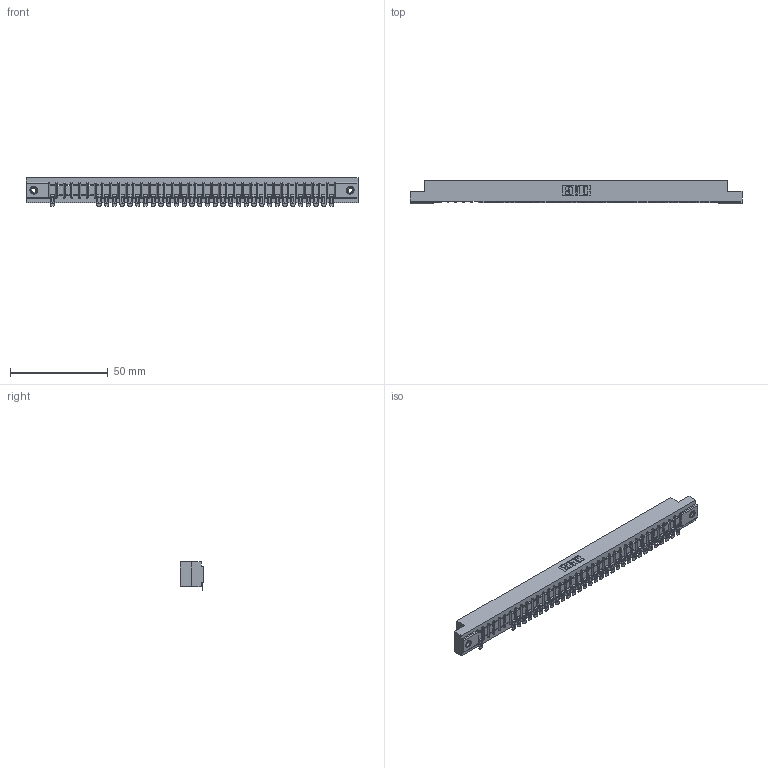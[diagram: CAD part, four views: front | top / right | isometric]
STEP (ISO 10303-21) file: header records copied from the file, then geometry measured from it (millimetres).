
FILE_DESCRIPTION (( 'STEP AP203' ), '1' );
FILE_NAME ('357-037-554-108.STEP', '2018-08-10T08:06:43', ( '' ), ( '' ), 'SwSTEP 2.0', 'SolidWorks 2016', '' );
FILE_SCHEMA (( 'CONFIG_CONTROL_DESIGN' ));
Length unit declared in the file: inch
Products named in the file (4): 357-037-554-108; 307 Part_.156 Dia Mounting Holes; 307-290-002_554; 345-250-001_345-250-003-102
Assembly tree (35 placements, depth 2):
  357-037-554-108
    307 Part_.156 Dia Mounting Holes
    307-290-002_554  x32
    345-250-001_345-250-003-102  x2
Bounding box: 169.62 x 12.01 x 14.52 mm (x, y, z)
Volume: 17974.7 mm3; surface area: 21707.2 mm2
Topology: 35 solids, 35 shells, 2908 faces, 8875 edges, 5806 vertices
Faces by surface type: plane 1634, cylinder 1182, sphere 76, cone 12, torus 4
Entity records: 34326 total; most frequent: CARTESIAN_POINT 5792, ORIENTED_EDGE 5780, DIRECTION 5640, EDGE_CURVE 2890, VECTOR 2204, LINE 2204, VERTEX_POINT 1870, AXIS2_PLACEMENT_3D 1718
